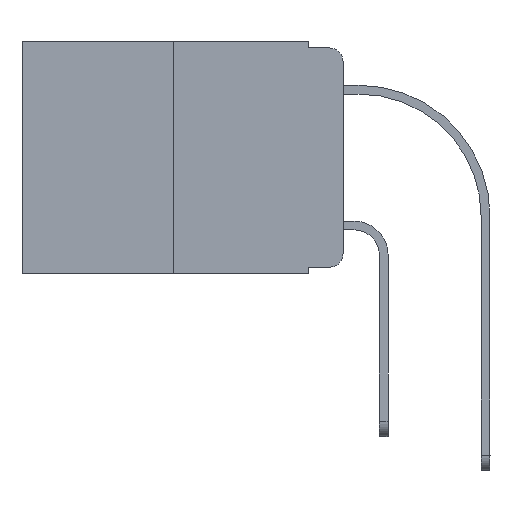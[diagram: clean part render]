
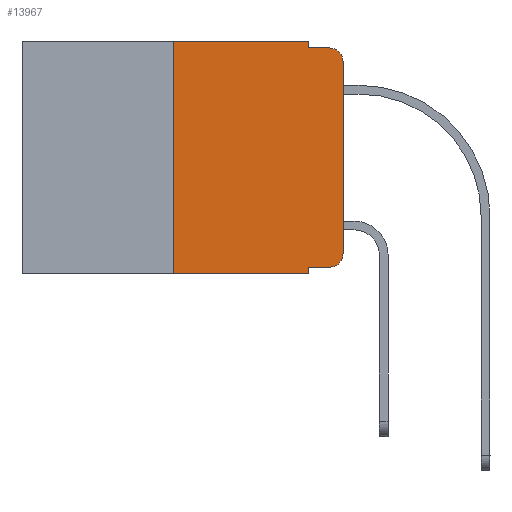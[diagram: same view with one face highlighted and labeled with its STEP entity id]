
A CAD part, left-side view. The second image highlights one B-rep face of the part: STEP entity #13967.
In plain terms, the highlighted planar face has unit normal (-1, 0, 0).
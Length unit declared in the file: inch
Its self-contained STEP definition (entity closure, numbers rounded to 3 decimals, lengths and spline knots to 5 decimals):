
#121 = LINE ( 'NONE', #21246, #16983 ) ;
#257 = VECTOR ( 'NONE', #11593, 39.37008 ) ;
#469 = EDGE_CURVE ( 'NONE', #9568, #20510, #552, .T. ) ;
#552 = LINE ( 'NONE', #2653, #4791 ) ;
#887 = DIRECTION ( 'NONE',  ( 0., 0., -1. ) ) ;
#2653 = CARTESIAN_POINT ( 'NONE',  ( 0., 0.473, 0. ) ) ;
#2748 = FACE_OUTER_BOUND ( 'NONE', #6660, .T. ) ;
#2984 = CARTESIAN_POINT ( 'NONE',  ( 0., 0.02, -0.313 ) ) ;
#4106 = VERTEX_POINT ( 'NONE', #9035 ) ;
#4187 = CIRCLE ( 'NONE', #11391, 0.02 ) ;
#4245 = CARTESIAN_POINT ( 'NONE',  ( 0., 0., -0.03 ) ) ;
#4517 = CARTESIAN_POINT ( 'NONE',  ( 0., 0.473, 0. ) ) ;
#4569 = ORIENTED_EDGE ( 'NONE', *, *, #14237, .F. ) ;
#4603 = CARTESIAN_POINT ( 'NONE',  ( 0., 0.02, -0.01 ) ) ;
#4791 = VECTOR ( 'NONE', #23172, 39.37008 ) ;
#5279 = VERTEX_POINT ( 'NONE', #24009 ) ;
#5696 = DIRECTION ( 'NONE',  ( 0., 0., -1. ) ) ;
#5750 = LINE ( 'NONE', #11412, #23252 ) ;
#6192 = DIRECTION ( 'NONE',  ( 0., -1., 0. ) ) ;
#6254 = VERTEX_POINT ( 'NONE', #13615 ) ;
#6528 = CARTESIAN_POINT ( 'NONE',  ( 0., 0.051, -0.01 ) ) ;
#6660 = EDGE_LOOP ( 'NONE', ( #22178, #12102, #8957, #19482, #12154, #4569, #14765, #9562, #9995, #11114 ) ) ;
#7051 = CARTESIAN_POINT ( 'NONE',  ( 0., 0.051, -0.333 ) ) ;
#7705 = CARTESIAN_POINT ( 'NONE',  ( 0., 0.051, 0. ) ) ;
#8039 = PLANE ( 'NONE',  #15773 ) ;
#8785 = CARTESIAN_POINT ( 'NONE',  ( 0., 0.051, 0. ) ) ;
#8957 = ORIENTED_EDGE ( 'NONE', *, *, #18344, .F. ) ;
#9016 = VECTOR ( 'NONE', #22278, 39.37008 ) ;
#9035 = CARTESIAN_POINT ( 'NONE',  ( 0., 0.051, -0.343 ) ) ;
#9562 = ORIENTED_EDGE ( 'NONE', *, *, #13483, .F. ) ;
#9568 = VERTEX_POINT ( 'NONE', #13689 ) ;
#9995 = ORIENTED_EDGE ( 'NONE', *, *, #15437, .T. ) ;
#10142 = CARTESIAN_POINT ( 'NONE',  ( 0., 0.051, -0.333 ) ) ;
#11114 = ORIENTED_EDGE ( 'NONE', *, *, #21035, .T. ) ;
#11391 = AXIS2_PLACEMENT_3D ( 'NONE', #15342, #16974, #5696 ) ;
#11412 = CARTESIAN_POINT ( 'NONE',  ( 0., 0., 0. ) ) ;
#11522 = DIRECTION ( 'NONE',  ( 0., 0., 1. ) ) ;
#11593 = DIRECTION ( 'NONE',  ( 0., 0., -1. ) ) ;
#12102 = ORIENTED_EDGE ( 'NONE', *, *, #20213, .T. ) ;
#12154 = ORIENTED_EDGE ( 'NONE', *, *, #469, .F. ) ;
#13037 = EDGE_CURVE ( 'NONE', #6254, #19575, #5750, .T. ) ;
#13212 = VERTEX_POINT ( 'NONE', #21977 ) ;
#13324 = VECTOR ( 'NONE', #17487, 39.37008 ) ;
#13354 = CARTESIAN_POINT ( 'NONE',  ( 0., 0.473, -0.343 ) ) ;
#13483 = EDGE_CURVE ( 'NONE', #20820, #4106, #18876, .T. ) ;
#13615 = CARTESIAN_POINT ( 'NONE',  ( 0., 0., -0.313 ) ) ;
#13689 = CARTESIAN_POINT ( 'NONE',  ( 0., 0.25, 0. ) ) ;
#13967 = ADVANCED_FACE ( 'NONE', ( #2748 ), #8039, .F. ) ;
#14237 = EDGE_CURVE ( 'NONE', #5279, #9568, #121, .T. ) ;
#14723 = AXIS2_PLACEMENT_3D ( 'NONE', #2984, #18250, #22491 ) ;
#14765 = ORIENTED_EDGE ( 'NONE', *, *, #16357, .T. ) ;
#15342 = CARTESIAN_POINT ( 'NONE',  ( 0., 0.02, -0.03 ) ) ;
#15437 = EDGE_CURVE ( 'NONE', #20820, #15595, #24147, .T. ) ;
#15485 = CARTESIAN_POINT ( 'NONE',  ( 0., 0.051, 0. ) ) ;
#15595 = VERTEX_POINT ( 'NONE', #21378 ) ;
#15773 = AXIS2_PLACEMENT_3D ( 'NONE', #4517, #18023, #887 ) ;
#16357 = EDGE_CURVE ( 'NONE', #5279, #4106, #22574, .T. ) ;
#16404 = EDGE_CURVE ( 'NONE', #20510, #13212, #19443, .T. ) ;
#16974 = DIRECTION ( 'NONE',  ( -1., 0., 0. ) ) ;
#16983 = VECTOR ( 'NONE', #11522, 39.37008 ) ;
#17487 = DIRECTION ( 'NONE',  ( 0., 0., -1. ) ) ;
#17797 = LINE ( 'NONE', #6528, #19518 ) ;
#18023 = DIRECTION ( 'NONE',  ( 1., 0., 0. ) ) ;
#18031 = DIRECTION ( 'NONE',  ( 0., -1., 0. ) ) ;
#18250 = DIRECTION ( 'NONE',  ( -1., 0., 0. ) ) ;
#18344 = EDGE_CURVE ( 'NONE', #13212, #19488, #17797, .T. ) ;
#18876 = LINE ( 'NONE', #15485, #13324 ) ;
#19015 = DIRECTION ( 'NONE',  ( 0., 0., 1. ) ) ;
#19443 = LINE ( 'NONE', #7705, #257 ) ;
#19482 = ORIENTED_EDGE ( 'NONE', *, *, #16404, .F. ) ;
#19488 = VERTEX_POINT ( 'NONE', #4603 ) ;
#19518 = VECTOR ( 'NONE', #18031, 39.37008 ) ;
#19575 = VERTEX_POINT ( 'NONE', #4245 ) ;
#20213 = EDGE_CURVE ( 'NONE', #19575, #19488, #4187, .T. ) ;
#20510 = VERTEX_POINT ( 'NONE', #8785 ) ;
#20820 = VERTEX_POINT ( 'NONE', #10142 ) ;
#21019 = VECTOR ( 'NONE', #6192, 39.37008 ) ;
#21035 = EDGE_CURVE ( 'NONE', #15595, #6254, #24265, .T. ) ;
#21246 = CARTESIAN_POINT ( 'NONE',  ( 0., 0.25, 0. ) ) ;
#21378 = CARTESIAN_POINT ( 'NONE',  ( 0., 0.02, -0.333 ) ) ;
#21977 = CARTESIAN_POINT ( 'NONE',  ( 0., 0.051, -0.01 ) ) ;
#22178 = ORIENTED_EDGE ( 'NONE', *, *, #13037, .T. ) ;
#22278 = DIRECTION ( 'NONE',  ( 0., -1., 0. ) ) ;
#22491 = DIRECTION ( 'NONE',  ( 0., 0., -1. ) ) ;
#22574 = LINE ( 'NONE', #13354, #21019 ) ;
#23172 = DIRECTION ( 'NONE',  ( 0., -1., 0. ) ) ;
#23252 = VECTOR ( 'NONE', #19015, 39.37008 ) ;
#24009 = CARTESIAN_POINT ( 'NONE',  ( 0., 0.25, -0.343 ) ) ;
#24147 = LINE ( 'NONE', #7051, #9016 ) ;
#24265 = CIRCLE ( 'NONE', #14723, 0.02 ) ;
